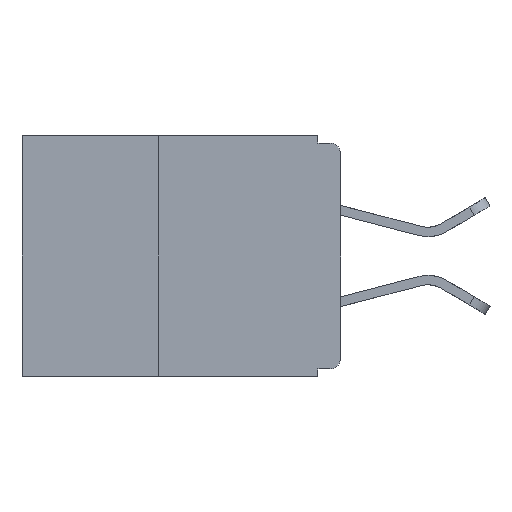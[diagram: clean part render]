
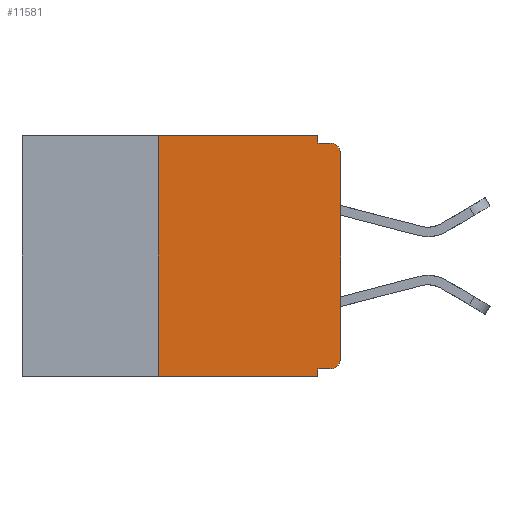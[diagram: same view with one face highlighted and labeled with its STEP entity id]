
A CAD part, left-side view. The second image highlights one B-rep face of the part: STEP entity #11581.
In plain terms, the highlighted planar face has unit normal (-1, 0, 0).
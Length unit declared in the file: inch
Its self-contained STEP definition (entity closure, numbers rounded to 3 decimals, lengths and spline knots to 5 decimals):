
#114 = VECTOR ( 'NONE', #8016, 39.37008 ) ;
#282 = CARTESIAN_POINT ( 'NONE',  ( 0., 0.031, -0.32 ) ) ;
#526 = VECTOR ( 'NONE', #13456, 39.37008 ) ;
#636 = DIRECTION ( 'NONE',  ( 0., 0., -1. ) ) ;
#930 = CARTESIAN_POINT ( 'NONE',  ( 0., 0., -0.305 ) ) ;
#1010 = LINE ( 'NONE', #7177, #3600 ) ;
#1172 = CARTESIAN_POINT ( 'NONE',  ( 0., 0., -0.025 ) ) ;
#1237 = VECTOR ( 'NONE', #636, 39.37008 ) ;
#1614 = EDGE_LOOP ( 'NONE', ( #5740, #10361, #10497, #10535, #10640, #10707, #11094, #11676, #12525, #10081 ) ) ;
#1617 = CARTESIAN_POINT ( 'NONE',  ( 0., 0., 0. ) ) ;
#1760 = CARTESIAN_POINT ( 'NONE',  ( 0., 0.437, 0. ) ) ;
#2501 = DIRECTION ( 'NONE',  ( 0., 0., 1. ) ) ;
#2575 = FACE_OUTER_BOUND ( 'NONE', #1614, .T. ) ;
#2754 = VECTOR ( 'NONE', #9476, 39.37008 ) ;
#3062 = VERTEX_POINT ( 'NONE', #282 ) ;
#3443 = EDGE_CURVE ( 'NONE', #13191, #3515, #1010, .T. ) ;
#3515 = VERTEX_POINT ( 'NONE', #10957 ) ;
#3600 = VECTOR ( 'NONE', #12362, 39.37008 ) ;
#3937 = DIRECTION ( 'NONE',  ( 0., 1., 0. ) ) ;
#4337 = EDGE_CURVE ( 'NONE', #9595, #8595, #7356, .T. ) ;
#4353 = CARTESIAN_POINT ( 'NONE',  ( 0., 0.25, -0.33 ) ) ;
#4550 = DIRECTION ( 'NONE',  ( -1., 0., 0. ) ) ;
#4604 = DIRECTION ( 'NONE',  ( 0., 0., -1. ) ) ;
#4605 = CARTESIAN_POINT ( 'NONE',  ( 0., 0.015, -0.305 ) ) ;
#4621 = DIRECTION ( 'NONE',  ( -1., 0., 0. ) ) ;
#4646 = CARTESIAN_POINT ( 'NONE',  ( 0., 0.015, -0.32 ) ) ;
#4662 = VECTOR ( 'NONE', #3937, 39.37008 ) ;
#5484 = VERTEX_POINT ( 'NONE', #4646 ) ;
#5740 = ORIENTED_EDGE ( 'NONE', *, *, #4337, .T. ) ;
#5840 = CARTESIAN_POINT ( 'NONE',  ( 0., 0.25, 0. ) ) ;
#5901 = LINE ( 'NONE', #7456, #114 ) ;
#6013 = CARTESIAN_POINT ( 'NONE',  ( 0., 0., -0.32 ) ) ;
#6315 = CARTESIAN_POINT ( 'NONE',  ( 0., 0.437, -0.33 ) ) ;
#6335 = EDGE_CURVE ( 'NONE', #9659, #11745, #5901, .T. ) ;
#6957 = LINE ( 'NONE', #13452, #1237 ) ;
#7032 = VECTOR ( 'NONE', #2501, 39.37008 ) ;
#7038 = VERTEX_POINT ( 'NONE', #11824 ) ;
#7156 = DIRECTION ( 'NONE',  ( 0., 0., -1. ) ) ;
#7177 = CARTESIAN_POINT ( 'NONE',  ( 0., 0., -0.01 ) ) ;
#7356 = LINE ( 'NONE', #1617, #7032 ) ;
#7381 = CARTESIAN_POINT ( 'NONE',  ( 0., 0.031, 0. ) ) ;
#7417 = LINE ( 'NONE', #6013, #4662 ) ;
#7456 = CARTESIAN_POINT ( 'NONE',  ( 0., 0.437, 0. ) ) ;
#8016 = DIRECTION ( 'NONE',  ( 0., -1., 0. ) ) ;
#8135 = DIRECTION ( 'NONE',  ( 0., 0., -1. ) ) ;
#8595 = VERTEX_POINT ( 'NONE', #1172 ) ;
#9180 = EDGE_CURVE ( 'NONE', #5484, #9595, #11877, .T. ) ;
#9362 = EDGE_CURVE ( 'NONE', #11745, #13191, #6957, .T. ) ;
#9476 = DIRECTION ( 'NONE',  ( 0., 0., 1. ) ) ;
#9595 = VERTEX_POINT ( 'NONE', #930 ) ;
#9659 = VERTEX_POINT ( 'NONE', #5840 ) ;
#10081 = ORIENTED_EDGE ( 'NONE', *, *, #9180, .T. ) ;
#10099 = LINE ( 'NONE', #12151, #12485 ) ;
#10165 = PLANE ( 'NONE',  #11507 ) ;
#10361 = ORIENTED_EDGE ( 'NONE', *, *, #13379, .T. ) ;
#10497 = ORIENTED_EDGE ( 'NONE', *, *, #3443, .F. ) ;
#10535 = ORIENTED_EDGE ( 'NONE', *, *, #9362, .F. ) ;
#10570 = EDGE_CURVE ( 'NONE', #12159, #7038, #11385, .T. ) ;
#10640 = ORIENTED_EDGE ( 'NONE', *, *, #6335, .F. ) ;
#10648 = EDGE_CURVE ( 'NONE', #12159, #9659, #13131, .T. ) ;
#10689 = CARTESIAN_POINT ( 'NONE',  ( 0., 0.015, -0.025 ) ) ;
#10707 = ORIENTED_EDGE ( 'NONE', *, *, #10648, .F. ) ;
#10957 = CARTESIAN_POINT ( 'NONE',  ( 0., 0.015, -0.01 ) ) ;
#11094 = ORIENTED_EDGE ( 'NONE', *, *, #10570, .T. ) ;
#11385 = LINE ( 'NONE', #6315, #526 ) ;
#11507 = AXIS2_PLACEMENT_3D ( 'NONE', #1760, #13234, #7156 ) ;
#11581 = ADVANCED_FACE ( 'NONE', ( #2575 ), #10165, .F. ) ;
#11676 = ORIENTED_EDGE ( 'NONE', *, *, #12533, .F. ) ;
#11701 = DIRECTION ( 'NONE',  ( 0., 0., -1. ) ) ;
#11745 = VERTEX_POINT ( 'NONE', #7381 ) ;
#11824 = CARTESIAN_POINT ( 'NONE',  ( 0., 0.031, -0.33 ) ) ;
#11877 = CIRCLE ( 'NONE', #12406, 0.015 ) ;
#12151 = CARTESIAN_POINT ( 'NONE',  ( 0., 0.031, -0.33 ) ) ;
#12159 = VERTEX_POINT ( 'NONE', #13179 ) ;
#12362 = DIRECTION ( 'NONE',  ( 0., -1., 0. ) ) ;
#12406 = AXIS2_PLACEMENT_3D ( 'NONE', #4605, #4621, #4604 ) ;
#12485 = VECTOR ( 'NONE', #8135, 39.37008 ) ;
#12514 = EDGE_CURVE ( 'NONE', #5484, #3062, #7417, .T. ) ;
#12525 = ORIENTED_EDGE ( 'NONE', *, *, #12514, .F. ) ;
#12533 = EDGE_CURVE ( 'NONE', #3062, #7038, #10099, .T. ) ;
#12787 = CIRCLE ( 'NONE', #13401, 0.015 ) ;
#13131 = LINE ( 'NONE', #4353, #2754 ) ;
#13179 = CARTESIAN_POINT ( 'NONE',  ( 0., 0.25, -0.33 ) ) ;
#13191 = VERTEX_POINT ( 'NONE', #13415 ) ;
#13234 = DIRECTION ( 'NONE',  ( 1., 0., 0. ) ) ;
#13379 = EDGE_CURVE ( 'NONE', #8595, #3515, #12787, .T. ) ;
#13401 = AXIS2_PLACEMENT_3D ( 'NONE', #10689, #4550, #11701 ) ;
#13415 = CARTESIAN_POINT ( 'NONE',  ( 0., 0.031, -0.01 ) ) ;
#13452 = CARTESIAN_POINT ( 'NONE',  ( 0., 0.031, 0. ) ) ;
#13456 = DIRECTION ( 'NONE',  ( 0., -1., 0. ) ) ;
